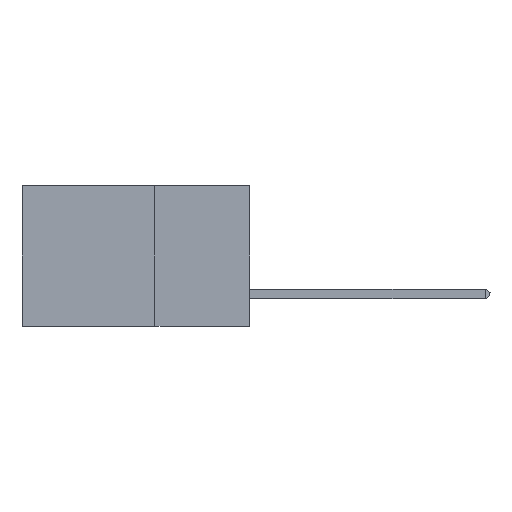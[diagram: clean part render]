
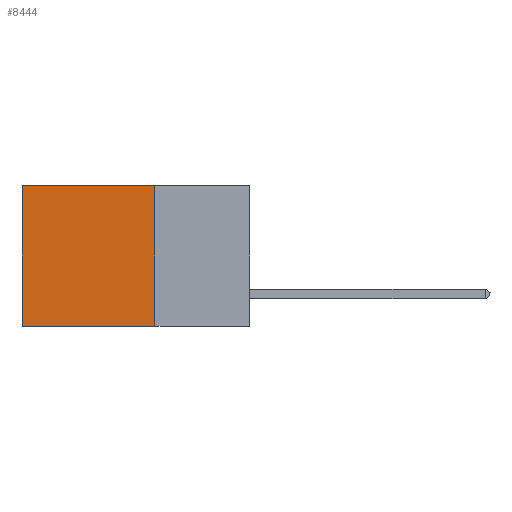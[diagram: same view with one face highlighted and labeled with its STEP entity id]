
A CAD part, left-side view. The second image highlights one B-rep face of the part: STEP entity #8444.
In plain terms, the highlighted planar face has unit normal (-1, 0, 0).
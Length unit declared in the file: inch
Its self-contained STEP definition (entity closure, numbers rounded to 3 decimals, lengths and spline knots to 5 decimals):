
#231 = DIRECTION ( 'NONE',  ( 0., 0., -1. ) ) ;
#759 = VERTEX_POINT ( 'NONE', #11485 ) ;
#1364 = VECTOR ( 'NONE', #11511, 39.37008 ) ;
#1385 = DIRECTION ( 'NONE',  ( 1., 0., 0. ) ) ;
#3491 = DIRECTION ( 'NONE',  ( 0., 0., -1. ) ) ;
#3492 = VECTOR ( 'NONE', #17648, 39.37008 ) ;
#3876 = CARTESIAN_POINT ( 'NONE',  ( 0.2875, 0.6, 0. ) ) ;
#4460 = VERTEX_POINT ( 'NONE', #14227 ) ;
#4843 = CARTESIAN_POINT ( 'NONE',  ( 0.2875, 0.25, 0. ) ) ;
#6272 = AXIS2_PLACEMENT_3D ( 'NONE', #23447, #1385, #3491 ) ;
#6915 = VECTOR ( 'NONE', #11360, 39.37008 ) ;
#8262 = EDGE_CURVE ( 'NONE', #759, #14386, #11480, .T. ) ;
#8444 = ADVANCED_FACE ( 'NONE', ( #14676 ), #8668, .F. ) ;
#8555 = EDGE_CURVE ( 'NONE', #16594, #4460, #12046, .T. ) ;
#8668 = PLANE ( 'NONE',  #6272 ) ;
#10923 = VECTOR ( 'NONE', #231, 39.37008 ) ;
#11360 = DIRECTION ( 'NONE',  ( 0., 1., 0. ) ) ;
#11480 = LINE ( 'NONE', #3876, #10923 ) ;
#11485 = CARTESIAN_POINT ( 'NONE',  ( 0.2875, 0.6, 0. ) ) ;
#11511 = DIRECTION ( 'NONE',  ( 0., 1., 0. ) ) ;
#12046 = LINE ( 'NONE', #4843, #3492 ) ;
#13175 = ORIENTED_EDGE ( 'NONE', *, *, #8555, .F. ) ;
#13767 = CARTESIAN_POINT ( 'NONE',  ( 0.2875, 0.25, 0. ) ) ;
#14227 = CARTESIAN_POINT ( 'NONE',  ( 0.2875, 0.25, -0.37 ) ) ;
#14386 = VERTEX_POINT ( 'NONE', #17798 ) ;
#14535 = EDGE_CURVE ( 'NONE', #4460, #14386, #21043, .T. ) ;
#14676 = FACE_OUTER_BOUND ( 'NONE', #19080, .T. ) ;
#15777 = LINE ( 'NONE', #16745, #6915 ) ;
#16486 = ORIENTED_EDGE ( 'NONE', *, *, #16710, .T. ) ;
#16594 = VERTEX_POINT ( 'NONE', #13767 ) ;
#16710 = EDGE_CURVE ( 'NONE', #16594, #759, #15777, .T. ) ;
#16745 = CARTESIAN_POINT ( 'NONE',  ( 0.2875, 0.25, 0. ) ) ;
#17259 = ORIENTED_EDGE ( 'NONE', *, *, #8262, .T. ) ;
#17648 = DIRECTION ( 'NONE',  ( 0., 0., -1. ) ) ;
#17798 = CARTESIAN_POINT ( 'NONE',  ( 0.2875, 0.6, -0.37 ) ) ;
#18817 = CARTESIAN_POINT ( 'NONE',  ( 0.2875, 0.25, -0.37 ) ) ;
#19080 = EDGE_LOOP ( 'NONE', ( #17259, #22738, #13175, #16486 ) ) ;
#21043 = LINE ( 'NONE', #18817, #1364 ) ;
#22738 = ORIENTED_EDGE ( 'NONE', *, *, #14535, .F. ) ;
#23447 = CARTESIAN_POINT ( 'NONE',  ( 0.2875, 0.25, 0. ) ) ;
